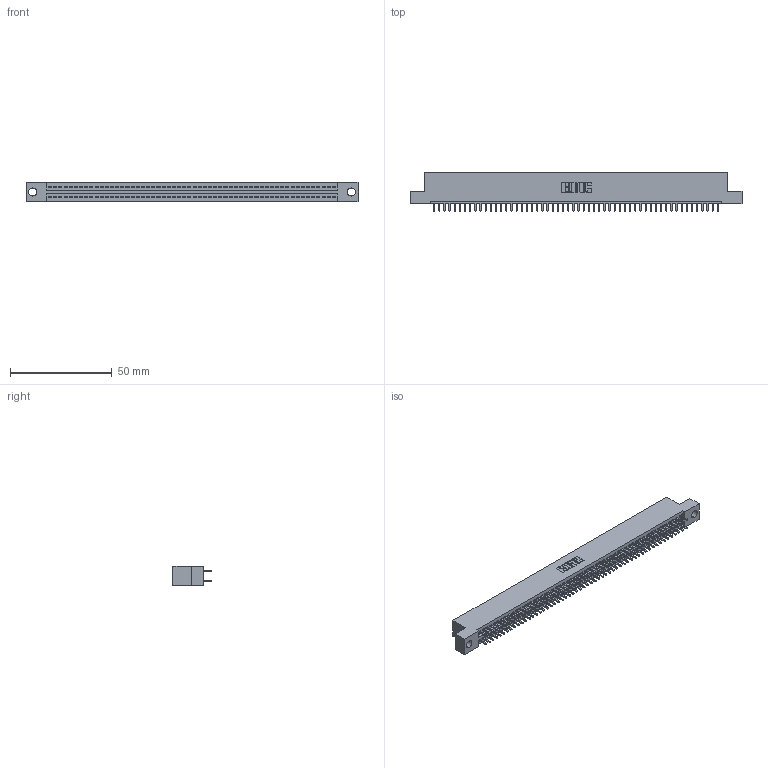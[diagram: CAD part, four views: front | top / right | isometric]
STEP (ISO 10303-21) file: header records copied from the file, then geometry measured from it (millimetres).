
FILE_DESCRIPTION (( 'STEP AP203' ), '1' );
FILE_NAME ('345-112-521-204.STEP', '2021-05-25T14:20:12', ( '' ), ( '' ), 'SwSTEP 2.0', 'SolidWorks 2020', '' );
FILE_SCHEMA (( 'CONFIG_CONTROL_DESIGN' ));
Length unit declared in the file: inch
Products named in the file (3): 345 Part_Flush Mounting Lugs - 0.156 Dia-TI; 345-292-001_345-293-121; 345-112-521-204
Assembly tree (113 placements, depth 2):
  345-112-521-204
    345 Part_Flush Mounting Lugs - 0.156 Dia-TI
    345-292-001_345-293-121  x112
Bounding box: 163.45 x 18.72 x 9.4 mm (x, y, z)
Volume: 15855.9 mm3; surface area: 23262.9 mm2
Topology: 113 solids, 113 shells, 5740 faces, 17065 edges, 11226 vertices
Faces by surface type: plane 3790, cylinder 1950
Entity records: 42491 total; most frequent: CARTESIAN_POINT 7114, ORIENTED_EDGE 7046, DIRECTION 6255, EDGE_CURVE 3523, LINE 3167, VECTOR 3167, VERTEX_POINT 2346, AXIS2_PLACEMENT_3D 1544
